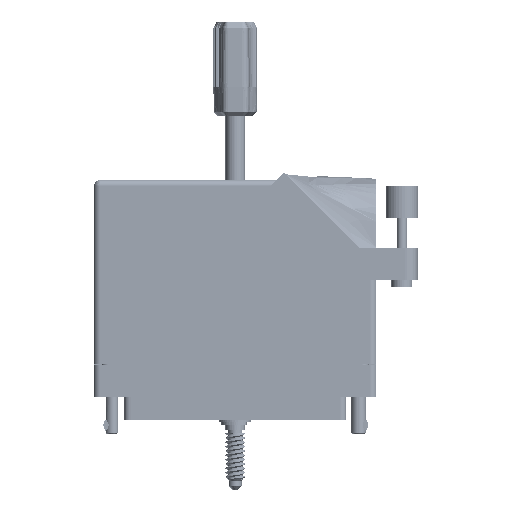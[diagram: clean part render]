
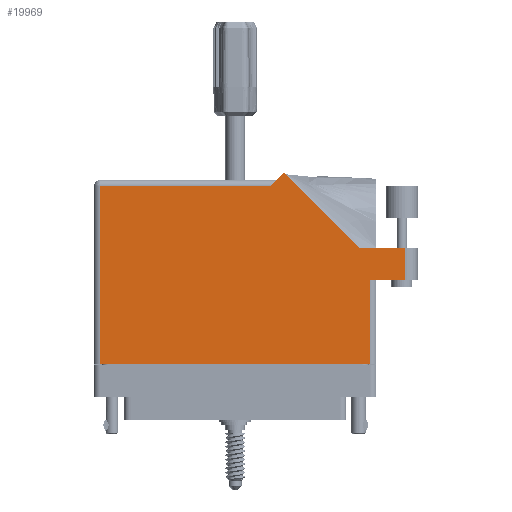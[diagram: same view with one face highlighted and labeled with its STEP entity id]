
A CAD part, front view. The second image highlights one B-rep face of the part: STEP entity #19969.
In plain terms, the highlighted face is planar.
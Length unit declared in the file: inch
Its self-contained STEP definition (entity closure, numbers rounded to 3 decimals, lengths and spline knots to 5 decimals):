
#2138 = VERTEX_POINT ( 'NONE', #80757 ) ;
#3065 = CARTESIAN_POINT ( 'NONE',  ( -1.359, -0.1, 0.617 ) ) ;
#4476 = VERTEX_POINT ( 'NONE', #12659 ) ;
#5392 = AXIS2_PLACEMENT_3D ( 'NONE', #18831, #56640, #70457 ) ;
#5462 = VECTOR ( 'NONE', #53089, 39.37008 ) ;
#6790 = EDGE_LOOP ( 'NONE', ( #31672, #78308, #37331, #68552, #80642, #31827, #31223, #15479, #74653 ) ) ;
#6967 = EDGE_CURVE ( 'NONE', #10496, #28014, #85330, .T. ) ;
#8608 = EDGE_CURVE ( 'NONE', #43469, #4476, #38238, .T. ) ;
#8871 = EDGE_CURVE ( 'NONE', #4476, #58623, #21980, .T. ) ;
#9787 = VECTOR ( 'NONE', #94913, 39.37008 ) ;
#10306 = DIRECTION ( 'NONE',  ( 1., 0., 0. ) ) ;
#10496 = VERTEX_POINT ( 'NONE', #78215 ) ;
#12659 = CARTESIAN_POINT ( 'NONE',  ( -1.297, -0.1, 0.617 ) ) ;
#13659 = CARTESIAN_POINT ( 'NONE',  ( -1.359, 1.613, 0.617 ) ) ;
#15479 = ORIENTED_EDGE ( 'NONE', *, *, #8871, .T. ) ;
#15984 = DIRECTION ( 'NONE',  ( -0.707, -0.707, 0. ) ) ;
#16606 = FACE_OUTER_BOUND ( 'NONE', #6790, .T. ) ;
#18162 = PLANE ( 'NONE',  #5392 ) ;
#18831 = CARTESIAN_POINT ( 'NONE',  ( -1.359, 1.675, 0.617 ) ) ;
#19969 = ADVANCED_FACE ( 'NONE', ( #16606 ), #18162, .F. ) ;
#21044 = EDGE_CURVE ( 'NONE', #41208, #33656, #88918, .T. ) ;
#21719 = LINE ( 'NONE', #94961, #59022 ) ;
#21980 = LINE ( 'NONE', #3065, #79211 ) ;
#22160 = LINE ( 'NONE', #13659, #84085 ) ;
#24466 = VECTOR ( 'NONE', #91750, 39.37008 ) ;
#25746 = VECTOR ( 'NONE', #47801, 39.37008 ) ;
#26070 = DIRECTION ( 'NONE',  ( 1., 0., 0. ) ) ;
#28014 = VERTEX_POINT ( 'NONE', #48978 ) ;
#28384 = CARTESIAN_POINT ( 'NONE',  ( 1.297, 0.715, 0.617 ) ) ;
#29054 = EDGE_CURVE ( 'NONE', #33656, #43469, #22160, .T. ) ;
#31223 = ORIENTED_EDGE ( 'NONE', *, *, #8608, .T. ) ;
#31672 = ORIENTED_EDGE ( 'NONE', *, *, #95914, .T. ) ;
#31827 = ORIENTED_EDGE ( 'NONE', *, *, #29054, .T. ) ;
#32326 = LINE ( 'NONE', #41635, #56819 ) ;
#33656 = VERTEX_POINT ( 'NONE', #84475 ) ;
#36389 = DIRECTION ( 'NONE',  ( -0.707, 0.707, 0. ) ) ;
#37331 = ORIENTED_EDGE ( 'NONE', *, *, #54796, .T. ) ;
#38238 = LINE ( 'NONE', #96672, #5462 ) ;
#39966 = CARTESIAN_POINT ( 'NONE',  ( 1.634, 1.022, 0.617 ) ) ;
#41208 = VERTEX_POINT ( 'NONE', #54356 ) ;
#41635 = CARTESIAN_POINT ( 'NONE',  ( 1.359, 0.715, 0.617 ) ) ;
#43469 = VERTEX_POINT ( 'NONE', #67968 ) ;
#45340 = CARTESIAN_POINT ( 'NONE',  ( 0.399, 1.675, 0.617 ) ) ;
#47801 = DIRECTION ( 'NONE',  ( 0., 1., 0. ) ) ;
#48978 = CARTESIAN_POINT ( 'NONE',  ( 1.634, 1.022, 0.617 ) ) ;
#53089 = DIRECTION ( 'NONE',  ( 0., -1., 0. ) ) ;
#54356 = CARTESIAN_POINT ( 'NONE',  ( 0.46971, 1.74571, 0.617 ) ) ;
#54796 = EDGE_CURVE ( 'NONE', #28014, #2138, #72315, .T. ) ;
#56640 = DIRECTION ( 'NONE',  ( 0., 0., -1. ) ) ;
#56819 = VECTOR ( 'NONE', #26070, 39.37008 ) ;
#58623 = VERTEX_POINT ( 'NONE', #91928 ) ;
#59022 = VECTOR ( 'NONE', #36389, 39.37008 ) ;
#61822 = EDGE_CURVE ( 'NONE', #2138, #41208, #21719, .T. ) ;
#67968 = CARTESIAN_POINT ( 'NONE',  ( -1.297, 1.613, 0.617 ) ) ;
#68552 = ORIENTED_EDGE ( 'NONE', *, *, #61822, .T. ) ;
#69000 = VECTOR ( 'NONE', #15984, 39.37008 ) ;
#70164 = CARTESIAN_POINT ( 'NONE',  ( 1.759, 1.022, 0.617 ) ) ;
#70457 = DIRECTION ( 'NONE',  ( -1., 0., 0. ) ) ;
#72160 = EDGE_CURVE ( 'NONE', #58623, #84890, #79943, .T. ) ;
#72315 = LINE ( 'NONE', #70164, #24466 ) ;
#74056 = DIRECTION ( 'NONE',  ( -1., 0., 0. ) ) ;
#74653 = ORIENTED_EDGE ( 'NONE', *, *, #72160, .T. ) ;
#78215 = CARTESIAN_POINT ( 'NONE',  ( 1.634, 0.715, 0.617 ) ) ;
#78308 = ORIENTED_EDGE ( 'NONE', *, *, #6967, .T. ) ;
#79211 = VECTOR ( 'NONE', #10306, 39.37008 ) ;
#79943 = LINE ( 'NONE', #88014, #9787 ) ;
#80642 = ORIENTED_EDGE ( 'NONE', *, *, #21044, .T. ) ;
#80757 = CARTESIAN_POINT ( 'NONE',  ( 1.19342, 1.022, 0.617 ) ) ;
#84085 = VECTOR ( 'NONE', #74056, 39.37008 ) ;
#84475 = CARTESIAN_POINT ( 'NONE',  ( 0.337, 1.613, 0.617 ) ) ;
#84890 = VERTEX_POINT ( 'NONE', #28384 ) ;
#85330 = LINE ( 'NONE', #39966, #25746 ) ;
#88014 = CARTESIAN_POINT ( 'NONE',  ( 1.297, 0.715, 0.617 ) ) ;
#88918 = LINE ( 'NONE', #45340, #69000 ) ;
#91750 = DIRECTION ( 'NONE',  ( -1., 0., 0. ) ) ;
#91928 = CARTESIAN_POINT ( 'NONE',  ( 1.297, -0.1, 0.617 ) ) ;
#94913 = DIRECTION ( 'NONE',  ( 0., 1., 0. ) ) ;
#94961 = CARTESIAN_POINT ( 'NONE',  ( 1.19342, 1.022, 0.617 ) ) ;
#95914 = EDGE_CURVE ( 'NONE', #84890, #10496, #32326, .T. ) ;
#96672 = CARTESIAN_POINT ( 'NONE',  ( -1.297, -0.1, 0.617 ) ) ;
